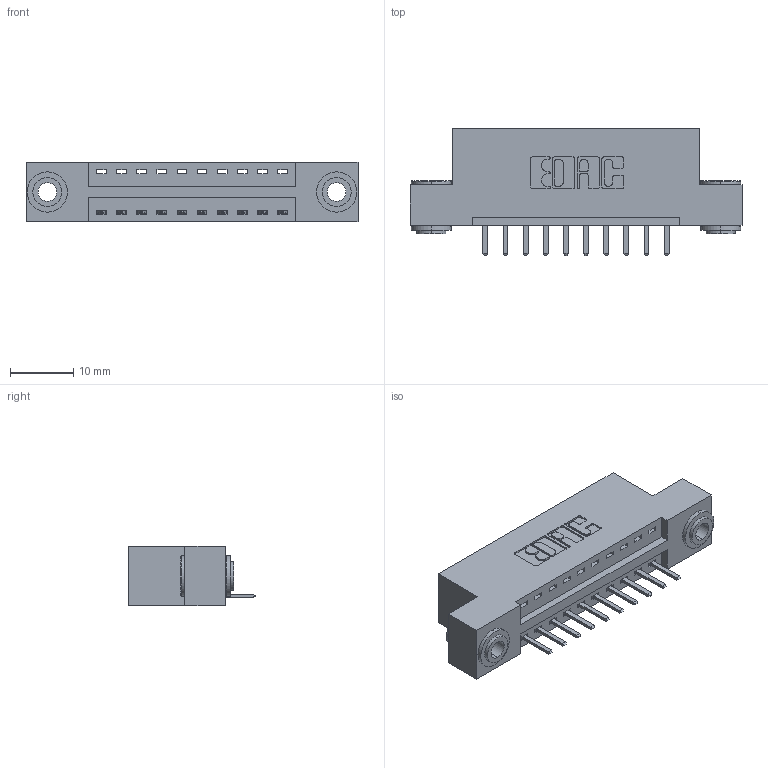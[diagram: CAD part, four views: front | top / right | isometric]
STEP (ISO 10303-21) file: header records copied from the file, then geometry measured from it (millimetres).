
FILE_DESCRIPTION (( 'STEP AP203' ), '1' );
FILE_NAME ('346-010-520-103.STEP', '2022-05-04T23:17:40', ( '' ), ( '' ), 'SwSTEP 2.0', 'SolidWorks 2020', '' );
FILE_SCHEMA (( 'CONFIG_CONTROL_DESIGN' ));
Length unit declared in the file: inch
Products named in the file (4): 346-010-520-103; 346 Part_Flush Mounting Lugs - 0.156 Dia-TH; 345-250-002_345-250-002-102; 345-292-001_345-293-120
Assembly tree (13 placements, depth 2):
  346-010-520-103
    346 Part_Flush Mounting Lugs - 0.156 Dia-TH
    345-292-001_345-293-120  x10
    345-250-002_345-250-002-102  x2
Bounding box: 52.32 x 20.02 x 9.4 mm (x, y, z)
Volume: 4760.6 mm3; surface area: 5760.3 mm2
Topology: 13 solids, 13 shells, 794 faces, 2281 edges, 1490 vertices
Faces by surface type: plane 520, cylinder 266, cone 8
Entity records: 11694 total; most frequent: CARTESIAN_POINT 2007, ORIENTED_EDGE 1930, DIRECTION 1827, EDGE_CURVE 965, LINE 765, VECTOR 765, VERTEX_POINT 638, AXIS2_PLACEMENT_3D 531
